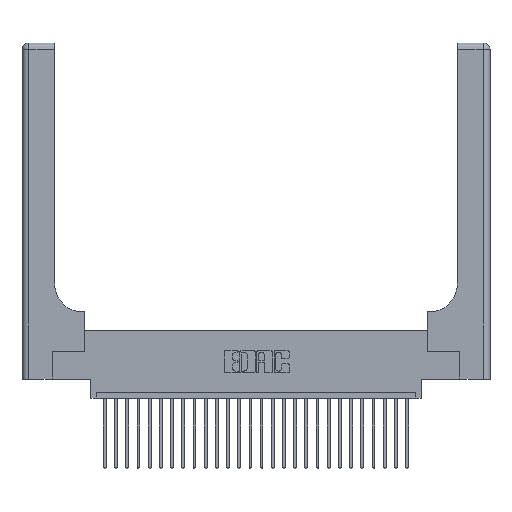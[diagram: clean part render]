
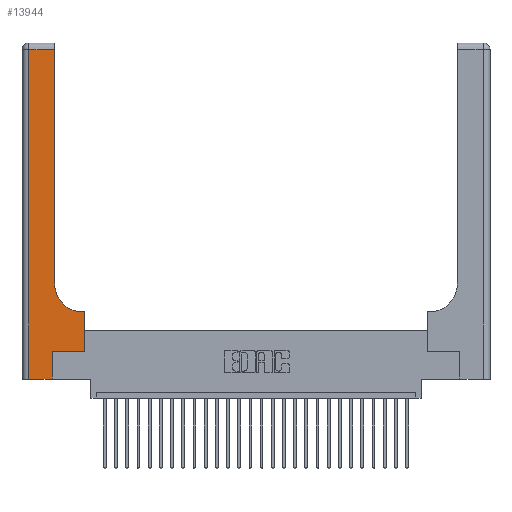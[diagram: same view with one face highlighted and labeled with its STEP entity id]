
A CAD part, top view. The second image highlights one B-rep face of the part: STEP entity #13944.
In plain terms, the highlighted planar face has unit normal (0, 0, 1).
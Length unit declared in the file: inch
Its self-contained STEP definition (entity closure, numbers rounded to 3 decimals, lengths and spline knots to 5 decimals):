
#348 = EDGE_CURVE ( 'NONE', #7456, #11352, #16382, .T. ) ;
#447 = CARTESIAN_POINT ( 'NONE',  ( 0.5585, 0.25, 0.37 ) ) ;
#741 = LINE ( 'NONE', #3721, #20204 ) ;
#880 = CARTESIAN_POINT ( 'NONE',  ( 0.5415, 0.6, 0.37 ) ) ;
#1124 = PLANE ( 'NONE',  #10225 ) ;
#1281 = EDGE_CURVE ( 'NONE', #22479, #27375, #2965, .T. ) ;
#2001 = DIRECTION ( 'NONE',  ( 0., -1., 0. ) ) ;
#2965 = LINE ( 'NONE', #15642, #16329 ) ;
#3328 = DIRECTION ( 'NONE',  ( -1., 0., 0. ) ) ;
#3430 = DIRECTION ( 'NONE',  ( 0., 0., -1. ) ) ;
#3721 = CARTESIAN_POINT ( 'NONE',  ( 0.269, 0., 0.37 ) ) ;
#4627 = DIRECTION ( 'NONE',  ( -1., 0., 0. ) ) ;
#4741 = LINE ( 'NONE', #21257, #27254 ) ;
#5163 = AXIS2_PLACEMENT_3D ( 'NONE', #13818, #10609, #12800 ) ;
#5534 = VECTOR ( 'NONE', #9462, 39.37008 ) ;
#6184 = VECTOR ( 'NONE', #15218, 39.37008 ) ;
#7456 = VERTEX_POINT ( 'NONE', #8712 ) ;
#7548 = CARTESIAN_POINT ( 'NONE',  ( 0.06, 0., 0.37 ) ) ;
#8712 = CARTESIAN_POINT ( 'NONE',  ( 0.5585, 0.6, 0.37 ) ) ;
#8979 = LINE ( 'NONE', #19860, #15815 ) ;
#9308 = ORIENTED_EDGE ( 'NONE', *, *, #348, .T. ) ;
#9462 = DIRECTION ( 'NONE',  ( 1., 0., 0. ) ) ;
#10209 = LINE ( 'NONE', #15170, #17697 ) ;
#10225 = AXIS2_PLACEMENT_3D ( 'NONE', #20775, #3430, #3328 ) ;
#10250 = FACE_OUTER_BOUND ( 'NONE', #11033, .T. ) ;
#10609 = DIRECTION ( 'NONE',  ( 0., 0., -1. ) ) ;
#11033 = EDGE_LOOP ( 'NONE', ( #16865, #26842, #11715, #20406, #25346, #13052, #25076, #9308, #26527 ) ) ;
#11352 = VERTEX_POINT ( 'NONE', #880 ) ;
#11715 = ORIENTED_EDGE ( 'NONE', *, *, #15972, .T. ) ;
#12174 = EDGE_CURVE ( 'NONE', #21068, #22007, #21560, .T. ) ;
#12338 = LINE ( 'NONE', #15121, #6184 ) ;
#12800 = DIRECTION ( 'NONE',  ( 1., 0., 0. ) ) ;
#13052 = ORIENTED_EDGE ( 'NONE', *, *, #12174, .T. ) ;
#13055 = EDGE_CURVE ( 'NONE', #22007, #7456, #12338, .T. ) ;
#13818 = CARTESIAN_POINT ( 'NONE',  ( 0.5415, 0.85, 0.37 ) ) ;
#13944 = ADVANCED_FACE ( 'NONE', ( #10250 ), #1124, .F. ) ;
#15121 = CARTESIAN_POINT ( 'NONE',  ( 0.5585, 0.25, 0.37 ) ) ;
#15170 = CARTESIAN_POINT ( 'NONE',  ( 0., 0., 0.37 ) ) ;
#15218 = DIRECTION ( 'NONE',  ( 0., 1., 0. ) ) ;
#15642 = CARTESIAN_POINT ( 'NONE',  ( 0., 2.94, 0.37 ) ) ;
#15815 = VECTOR ( 'NONE', #22696, 39.37008 ) ;
#15972 = EDGE_CURVE ( 'NONE', #27375, #22813, #4741, .T. ) ;
#16329 = VECTOR ( 'NONE', #4627, 39.37008 ) ;
#16382 = LINE ( 'NONE', #26010, #22797 ) ;
#16823 = CIRCLE ( 'NONE', #5163, 0.25 ) ;
#16865 = ORIENTED_EDGE ( 'NONE', *, *, #20436, .T. ) ;
#17139 = EDGE_CURVE ( 'NONE', #22813, #18525, #10209, .T. ) ;
#17339 = CARTESIAN_POINT ( 'NONE',  ( 0.269, 0.25, 0.37 ) ) ;
#17542 = DIRECTION ( 'NONE',  ( -1., 0., 0. ) ) ;
#17697 = VECTOR ( 'NONE', #23712, 39.37008 ) ;
#18525 = VERTEX_POINT ( 'NONE', #27750 ) ;
#18714 = DIRECTION ( 'NONE',  ( 0., 1., 0. ) ) ;
#18810 = CARTESIAN_POINT ( 'NONE',  ( 0.2915, 0.85, 0.37 ) ) ;
#19768 = EDGE_CURVE ( 'NONE', #18525, #21068, #741, .T. ) ;
#19860 = CARTESIAN_POINT ( 'NONE',  ( 0.2915, 3., 0.37 ) ) ;
#20204 = VECTOR ( 'NONE', #18714, 39.37008 ) ;
#20406 = ORIENTED_EDGE ( 'NONE', *, *, #17139, .T. ) ;
#20436 = EDGE_CURVE ( 'NONE', #20953, #22479, #8979, .T. ) ;
#20756 = EDGE_CURVE ( 'NONE', #11352, #20953, #16823, .T. ) ;
#20775 = CARTESIAN_POINT ( 'NONE',  ( 0., 3., 0.37 ) ) ;
#20844 = CARTESIAN_POINT ( 'NONE',  ( 0.06, 2.94, 0.37 ) ) ;
#20953 = VERTEX_POINT ( 'NONE', #18810 ) ;
#21068 = VERTEX_POINT ( 'NONE', #17339 ) ;
#21257 = CARTESIAN_POINT ( 'NONE',  ( 0.06, 3., 0.37 ) ) ;
#21560 = LINE ( 'NONE', #26684, #5534 ) ;
#22007 = VERTEX_POINT ( 'NONE', #447 ) ;
#22479 = VERTEX_POINT ( 'NONE', #24229 ) ;
#22696 = DIRECTION ( 'NONE',  ( 0., 1., 0. ) ) ;
#22797 = VECTOR ( 'NONE', #17542, 39.37008 ) ;
#22813 = VERTEX_POINT ( 'NONE', #7548 ) ;
#23712 = DIRECTION ( 'NONE',  ( 1., 0., 0. ) ) ;
#24229 = CARTESIAN_POINT ( 'NONE',  ( 0.2915, 2.94, 0.37 ) ) ;
#25076 = ORIENTED_EDGE ( 'NONE', *, *, #13055, .T. ) ;
#25346 = ORIENTED_EDGE ( 'NONE', *, *, #19768, .T. ) ;
#26010 = CARTESIAN_POINT ( 'NONE',  ( 0.2915, 0.6, 0.37 ) ) ;
#26527 = ORIENTED_EDGE ( 'NONE', *, *, #20756, .T. ) ;
#26684 = CARTESIAN_POINT ( 'NONE',  ( 0.269, 0.25, 0.37 ) ) ;
#26842 = ORIENTED_EDGE ( 'NONE', *, *, #1281, .T. ) ;
#27254 = VECTOR ( 'NONE', #2001, 39.37008 ) ;
#27375 = VERTEX_POINT ( 'NONE', #20844 ) ;
#27750 = CARTESIAN_POINT ( 'NONE',  ( 0.269, 0., 0.37 ) ) ;
